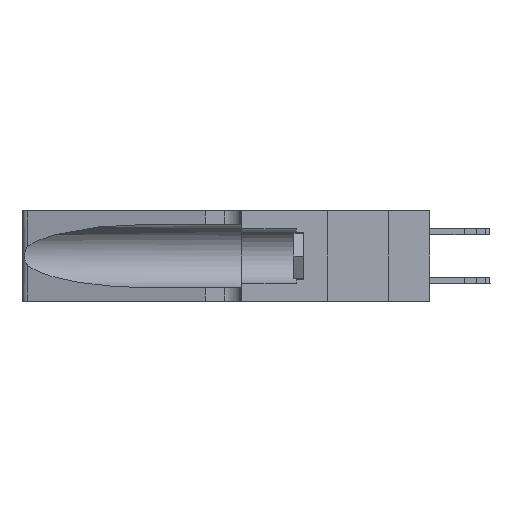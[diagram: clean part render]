
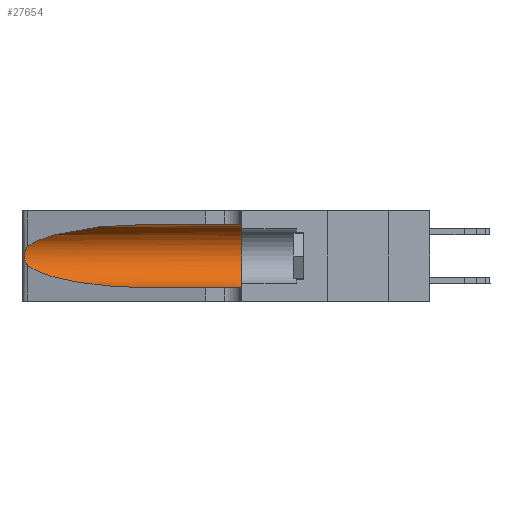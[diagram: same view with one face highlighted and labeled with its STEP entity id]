
A CAD part, left-side view. The second image highlights one B-rep face of the part: STEP entity #27654.
In plain terms, the highlighted cylindrical face has radius 3.308 mm (diameter 6.617 mm), a partial arc.
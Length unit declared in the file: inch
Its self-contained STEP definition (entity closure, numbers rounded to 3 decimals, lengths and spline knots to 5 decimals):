
#623 = CARTESIAN_POINT ( 'NONE',  ( 0.25639, 1.23184, 0.21858 ) ) ;
#664 = VERTEX_POINT ( 'NONE', #22044 ) ;
#1259 = CARTESIAN_POINT ( 'NONE',  ( 0.26018, 1.23835, 0.19895 ) ) ;
#1513 = VERTEX_POINT ( 'NONE', #17368 ) ;
#1887 = CARTESIAN_POINT ( 'NONE',  ( 0.1305, 1.61858, 0.31525 ) ) ;
#2017 = EDGE_CURVE ( 'NONE', #17960, #5605, #31484, .T. ) ;
#2597 = CARTESIAN_POINT ( 'NONE',  ( 0.1305, 0.35, 0.185 ) ) ;
#3826 = CARTESIAN_POINT ( 'NONE',  ( 0.1305, 0.35, 0.31525 ) ) ;
#4025 = DIRECTION ( 'NONE',  ( 0., 0., -1. ) ) ;
#4212 = ORIENTED_EDGE ( 'NONE', *, *, #30033, .T. ) ;
#5079 =( BOUNDED_CURVE ( )  B_SPLINE_CURVE ( 3, ( #16134, #7992, #18942, #14618 ),
 .UNSPECIFIED., .F., .F. ) 
 B_SPLINE_CURVE_WITH_KNOTS ( ( 4, 4 ),
 ( 1.5708, 2.84003 ),
 .UNSPECIFIED. ) 
 CURVE ( )  GEOMETRIC_REPRESENTATION_ITEM ( )  RATIONAL_B_SPLINE_CURVE ( ( 1., 0.87, 0.87, 1. ) ) 
 REPRESENTATION_ITEM ( '' )  );
#5605 = VERTEX_POINT ( 'NONE', #3826 ) ;
#6082 = EDGE_CURVE ( 'NONE', #17960, #23035, #5079, .T. ) ;
#6544 =( BOUNDED_CURVE ( )  B_SPLINE_CURVE ( 3, ( #17534, #23067, #13116, #30113 ),
 .UNSPECIFIED., .F., .T. ) 
 B_SPLINE_CURVE_WITH_KNOTS ( ( 4, 4 ),
 ( 3.44316, 4.71239 ),
 .UNSPECIFIED. ) 
 CURVE ( )  GEOMETRIC_REPRESENTATION_ITEM ( )  RATIONAL_B_SPLINE_CURVE ( ( 1., 0.87, 0.87, 1. ) ) 
 REPRESENTATION_ITEM ( '' )  );
#7388 = CYLINDRICAL_SURFACE ( 'NONE', #29621, 0.13025 ) ;
#7684 = ORIENTED_EDGE ( 'NONE', *, *, #15911, .F. ) ;
#7992 = CARTESIAN_POINT ( 'NONE',  ( 0.18966, 0.96281, 0.31525 ) ) ;
#8804 = ORIENTED_EDGE ( 'NONE', *, *, #6082, .T. ) ;
#9171 = CARTESIAN_POINT ( 'NONE',  ( 0.25487, 1.22718, 0.14631 ) ) ;
#9765 = B_SPLINE_CURVE_WITH_KNOTS ( 'NONE', 3,
 ( #16536, #21913, #623, #14679, #25180, #1259, #30932, #11838, #19913, #30815, #20152, #17116, #30575, #9171 ),
 .UNSPECIFIED., .F., .F.,
 ( 4, 2, 2, 2, 2, 2, 4 ),
 ( 0., 0.00027, 0.00053, 0.00107, 0.0016, 0.00187, 0.00214 ),
 .UNSPECIFIED. ) ;
#11838 = CARTESIAN_POINT ( 'NONE',  ( 0.26075, 1.23896, 0.178 ) ) ;
#11917 = LINE ( 'NONE', #32912, #21551 ) ;
#12847 = ORIENTED_EDGE ( 'NONE', *, *, #22048, .T. ) ;
#13116 = CARTESIAN_POINT ( 'NONE',  ( 0.18966, 0.96281, 0.05475 ) ) ;
#14120 = EDGE_CURVE ( 'NONE', #30038, #1513, #6544, .T. ) ;
#14618 = CARTESIAN_POINT ( 'NONE',  ( 0.25487, 1.22718, 0.22369 ) ) ;
#14679 = CARTESIAN_POINT ( 'NONE',  ( 0.25787, 1.23484, 0.2124 ) ) ;
#15911 = EDGE_CURVE ( 'NONE', #5605, #664, #29764, .T. ) ;
#16071 = DIRECTION ( 'NONE',  ( 0., 0., 1. ) ) ;
#16134 = CARTESIAN_POINT ( 'NONE',  ( 0.1305, 0.72297, 0.31525 ) ) ;
#16536 = CARTESIAN_POINT ( 'NONE',  ( 0.25487, 1.22718, 0.22369 ) ) ;
#16798 = CARTESIAN_POINT ( 'NONE',  ( 0.1305, 1.61858, 0.185 ) ) ;
#17116 = CARTESIAN_POINT ( 'NONE',  ( 0.25639, 1.23186, 0.15144 ) ) ;
#17368 = CARTESIAN_POINT ( 'NONE',  ( 0.1305, 0.72297, 0.05475 ) ) ;
#17534 = CARTESIAN_POINT ( 'NONE',  ( 0.25487, 1.22718, 0.14631 ) ) ;
#17960 = VERTEX_POINT ( 'NONE', #25539 ) ;
#18942 = CARTESIAN_POINT ( 'NONE',  ( 0.2373, 1.15595, 0.28018 ) ) ;
#19274 = VECTOR ( 'NONE', #32550, 39.37008 ) ;
#19580 = DIRECTION ( 'NONE',  ( 0., -1., 0. ) ) ;
#19913 = CARTESIAN_POINT ( 'NONE',  ( 0.26017, 1.23833, 0.17102 ) ) ;
#20152 = CARTESIAN_POINT ( 'NONE',  ( 0.25789, 1.23486, 0.15765 ) ) ;
#21551 = VECTOR ( 'NONE', #32573, 39.37008 ) ;
#21913 = CARTESIAN_POINT ( 'NONE',  ( 0.25555, 1.22994, 0.2215 ) ) ;
#21965 = FACE_OUTER_BOUND ( 'NONE', #24851, .T. ) ;
#22044 = CARTESIAN_POINT ( 'NONE',  ( 0.1305, 0.35, 0.05475 ) ) ;
#22048 = EDGE_CURVE ( 'NONE', #1513, #664, #11917, .T. ) ;
#23035 = VERTEX_POINT ( 'NONE', #31418 ) ;
#23067 = CARTESIAN_POINT ( 'NONE',  ( 0.2373, 1.15595, 0.08982 ) ) ;
#23950 = DIRECTION ( 'NONE',  ( 0., 1., 0. ) ) ;
#24851 = EDGE_LOOP ( 'NONE', ( #8804, #4212, #28392, #12847, #7684, #34124 ) ) ;
#25180 = CARTESIAN_POINT ( 'NONE',  ( 0.25854, 1.2359, 0.20912 ) ) ;
#25539 = CARTESIAN_POINT ( 'NONE',  ( 0.1305, 0.72297, 0.31525 ) ) ;
#27654 = ADVANCED_FACE ( 'NONE', ( #21965 ), #7388, .F. ) ;
#28195 = AXIS2_PLACEMENT_3D ( 'NONE', #2597, #23950, #16071 ) ;
#28392 = ORIENTED_EDGE ( 'NONE', *, *, #14120, .T. ) ;
#29621 = AXIS2_PLACEMENT_3D ( 'NONE', #16798, #19580, #4025 ) ;
#29764 = CIRCLE ( 'NONE', #28195, 0.13025 ) ;
#30033 = EDGE_CURVE ( 'NONE', #23035, #30038, #9765, .T. ) ;
#30038 = VERTEX_POINT ( 'NONE', #33111 ) ;
#30113 = CARTESIAN_POINT ( 'NONE',  ( 0.1305, 0.72297, 0.05475 ) ) ;
#30575 = CARTESIAN_POINT ( 'NONE',  ( 0.25555, 1.22993, 0.14849 ) ) ;
#30815 = CARTESIAN_POINT ( 'NONE',  ( 0.25856, 1.23593, 0.16098 ) ) ;
#30932 = CARTESIAN_POINT ( 'NONE',  ( 0.26075, 1.23896, 0.19203 ) ) ;
#31418 = CARTESIAN_POINT ( 'NONE',  ( 0.25487, 1.22718, 0.22369 ) ) ;
#31484 = LINE ( 'NONE', #1887, #19274 ) ;
#32550 = DIRECTION ( 'NONE',  ( 0., -1., 0. ) ) ;
#32573 = DIRECTION ( 'NONE',  ( 0., -1., 0. ) ) ;
#32912 = CARTESIAN_POINT ( 'NONE',  ( 0.1305, 1.61858, 0.05475 ) ) ;
#33111 = CARTESIAN_POINT ( 'NONE',  ( 0.25487, 1.22718, 0.14631 ) ) ;
#34124 = ORIENTED_EDGE ( 'NONE', *, *, #2017, .F. ) ;
